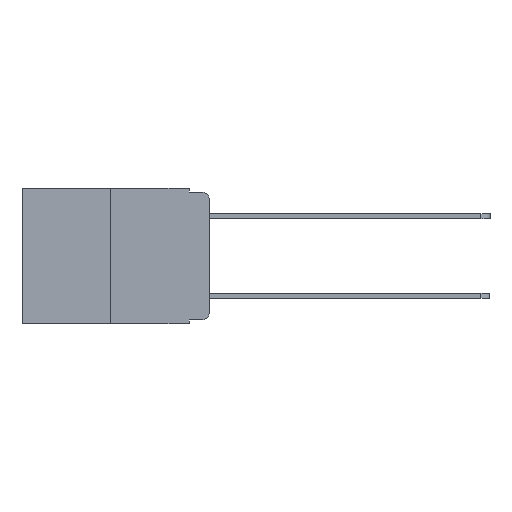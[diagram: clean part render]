
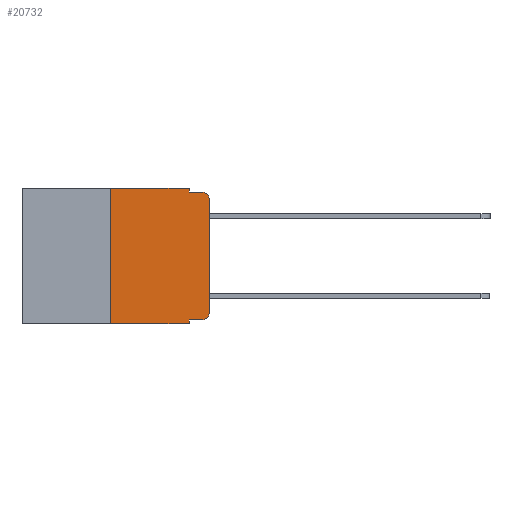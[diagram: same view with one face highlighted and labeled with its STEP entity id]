
A CAD part, left-side view. The second image highlights one B-rep face of the part: STEP entity #20732.
In plain terms, the highlighted planar face has unit normal (-1, 0, 0).
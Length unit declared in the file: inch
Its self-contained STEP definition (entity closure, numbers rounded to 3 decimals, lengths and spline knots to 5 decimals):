
#108 = CARTESIAN_POINT ( 'NONE',  ( 0., 0.25, 0. ) ) ;
#357 = DIRECTION ( 'NONE',  ( 0., 0., -1. ) ) ;
#524 = CARTESIAN_POINT ( 'NONE',  ( 0., 0.02, -0.333 ) ) ;
#548 = CIRCLE ( 'NONE', #2688, 0.02 ) ;
#569 = CARTESIAN_POINT ( 'NONE',  ( 0., 0.051, -0.333 ) ) ;
#630 = LINE ( 'NONE', #108, #9922 ) ;
#935 = CARTESIAN_POINT ( 'NONE',  ( 0., 0.473, -0.343 ) ) ;
#1455 = EDGE_CURVE ( 'NONE', #9525, #10731, #2165, .T. ) ;
#1802 = CARTESIAN_POINT ( 'NONE',  ( 0., 0., 0. ) ) ;
#1960 = DIRECTION ( 'NONE',  ( 0., 0., 1. ) ) ;
#2165 = LINE ( 'NONE', #19392, #7709 ) ;
#2428 = CARTESIAN_POINT ( 'NONE',  ( 0., 0.051, 0. ) ) ;
#2688 = AXIS2_PLACEMENT_3D ( 'NONE', #4754, #17564, #6644 ) ;
#2799 = DIRECTION ( 'NONE',  ( 0., -1., 0. ) ) ;
#2802 = ORIENTED_EDGE ( 'NONE', *, *, #6085, .F. ) ;
#3484 = VERTEX_POINT ( 'NONE', #23518 ) ;
#3894 = VERTEX_POINT ( 'NONE', #19220 ) ;
#4008 = CARTESIAN_POINT ( 'NONE',  ( 0., 0.051, -0.343 ) ) ;
#4144 = LINE ( 'NONE', #22145, #13356 ) ;
#4209 = DIRECTION ( 'NONE',  ( 0., 0., -1. ) ) ;
#4232 = CARTESIAN_POINT ( 'NONE',  ( 0., 0.051, -0.01 ) ) ;
#4314 = VECTOR ( 'NONE', #2799, 39.37008 ) ;
#4754 = CARTESIAN_POINT ( 'NONE',  ( 0., 0.02, -0.313 ) ) ;
#4887 = DIRECTION ( 'NONE',  ( 0., -1., 0. ) ) ;
#4936 = ORIENTED_EDGE ( 'NONE', *, *, #22855, .T. ) ;
#5944 = CARTESIAN_POINT ( 'NONE',  ( 0., 0.25, -0.343 ) ) ;
#6085 = EDGE_CURVE ( 'NONE', #10033, #17762, #4144, .T. ) ;
#6644 = DIRECTION ( 'NONE',  ( 0., 0., -1. ) ) ;
#7351 = ORIENTED_EDGE ( 'NONE', *, *, #8423, .F. ) ;
#7709 = VECTOR ( 'NONE', #19315, 39.37008 ) ;
#7719 = ORIENTED_EDGE ( 'NONE', *, *, #12993, .F. ) ;
#7912 = CARTESIAN_POINT ( 'NONE',  ( 0., 0.473, 0. ) ) ;
#7941 = DIRECTION ( 'NONE',  ( -1., 0., 0. ) ) ;
#8254 = FACE_OUTER_BOUND ( 'NONE', #20068, .T. ) ;
#8423 = EDGE_CURVE ( 'NONE', #19778, #10033, #12668, .T. ) ;
#8822 = VERTEX_POINT ( 'NONE', #5944 ) ;
#8879 = VERTEX_POINT ( 'NONE', #524 ) ;
#9139 = CARTESIAN_POINT ( 'NONE',  ( 0., 0.051, -0.333 ) ) ;
#9525 = VERTEX_POINT ( 'NONE', #569 ) ;
#9690 = EDGE_CURVE ( 'NONE', #8879, #3484, #548, .T. ) ;
#9922 = VECTOR ( 'NONE', #1960, 39.37008 ) ;
#10033 = VERTEX_POINT ( 'NONE', #2428 ) ;
#10682 = ORIENTED_EDGE ( 'NONE', *, *, #10753, .T. ) ;
#10731 = VERTEX_POINT ( 'NONE', #4008 ) ;
#10753 = EDGE_CURVE ( 'NONE', #16994, #3894, #11211, .T. ) ;
#10978 = DIRECTION ( 'NONE',  ( 0., -1., 0. ) ) ;
#11211 = CIRCLE ( 'NONE', #18472, 0.02 ) ;
#11568 = VECTOR ( 'NONE', #13478, 39.37008 ) ;
#12117 = VECTOR ( 'NONE', #4887, 39.37008 ) ;
#12668 = LINE ( 'NONE', #19438, #12117 ) ;
#12813 = DIRECTION ( 'NONE',  ( 0., 0., 1. ) ) ;
#12991 = ORIENTED_EDGE ( 'NONE', *, *, #22725, .F. ) ;
#12993 = EDGE_CURVE ( 'NONE', #8822, #19778, #630, .T. ) ;
#13172 = VECTOR ( 'NONE', #10978, 39.37008 ) ;
#13356 = VECTOR ( 'NONE', #357, 39.37008 ) ;
#13478 = DIRECTION ( 'NONE',  ( 0., -1., 0. ) ) ;
#14535 = ORIENTED_EDGE ( 'NONE', *, *, #17394, .T. ) ;
#14896 = VECTOR ( 'NONE', #12813, 39.37008 ) ;
#15195 = DIRECTION ( 'NONE',  ( 1., 0., 0. ) ) ;
#16406 = LINE ( 'NONE', #4232, #11568 ) ;
#16597 = AXIS2_PLACEMENT_3D ( 'NONE', #7912, #15195, #4209 ) ;
#16994 = VERTEX_POINT ( 'NONE', #20585 ) ;
#17394 = EDGE_CURVE ( 'NONE', #3484, #16994, #19641, .T. ) ;
#17555 = CARTESIAN_POINT ( 'NONE',  ( 0., 0.051, -0.01 ) ) ;
#17564 = DIRECTION ( 'NONE',  ( -1., 0., 0. ) ) ;
#17762 = VERTEX_POINT ( 'NONE', #17555 ) ;
#18472 = AXIS2_PLACEMENT_3D ( 'NONE', #18764, #7941, #20528 ) ;
#18537 = LINE ( 'NONE', #9139, #13172 ) ;
#18589 = EDGE_CURVE ( 'NONE', #9525, #8879, #18537, .T. ) ;
#18764 = CARTESIAN_POINT ( 'NONE',  ( 0., 0.02, -0.03 ) ) ;
#18872 = LINE ( 'NONE', #935, #4314 ) ;
#19219 = CARTESIAN_POINT ( 'NONE',  ( 0., 0.25, 0. ) ) ;
#19220 = CARTESIAN_POINT ( 'NONE',  ( 0., 0.02, -0.01 ) ) ;
#19315 = DIRECTION ( 'NONE',  ( 0., 0., -1. ) ) ;
#19392 = CARTESIAN_POINT ( 'NONE',  ( 0., 0.051, 0. ) ) ;
#19438 = CARTESIAN_POINT ( 'NONE',  ( 0., 0.473, 0. ) ) ;
#19641 = LINE ( 'NONE', #1802, #14896 ) ;
#19778 = VERTEX_POINT ( 'NONE', #19219 ) ;
#20068 = EDGE_LOOP ( 'NONE', ( #14535, #10682, #12991, #2802, #7351, #7719, #4936, #22918, #22807, #23238 ) ) ;
#20494 = PLANE ( 'NONE',  #16597 ) ;
#20528 = DIRECTION ( 'NONE',  ( 0., 0., -1. ) ) ;
#20585 = CARTESIAN_POINT ( 'NONE',  ( 0., 0., -0.03 ) ) ;
#20732 = ADVANCED_FACE ( 'NONE', ( #8254 ), #20494, .F. ) ;
#22145 = CARTESIAN_POINT ( 'NONE',  ( 0., 0.051, 0. ) ) ;
#22725 = EDGE_CURVE ( 'NONE', #17762, #3894, #16406, .T. ) ;
#22807 = ORIENTED_EDGE ( 'NONE', *, *, #18589, .T. ) ;
#22855 = EDGE_CURVE ( 'NONE', #8822, #10731, #18872, .T. ) ;
#22918 = ORIENTED_EDGE ( 'NONE', *, *, #1455, .F. ) ;
#23238 = ORIENTED_EDGE ( 'NONE', *, *, #9690, .T. ) ;
#23518 = CARTESIAN_POINT ( 'NONE',  ( 0., 0., -0.313 ) ) ;
